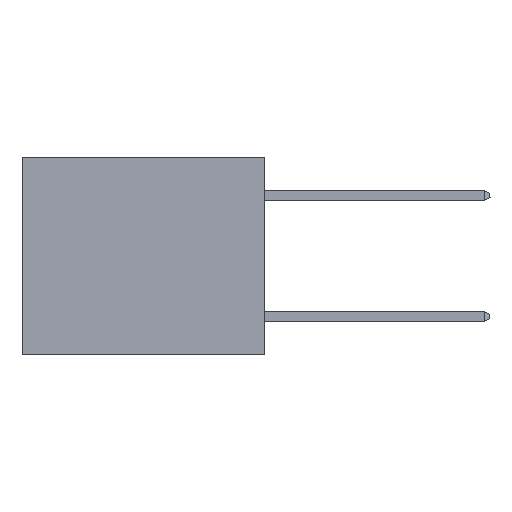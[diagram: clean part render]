
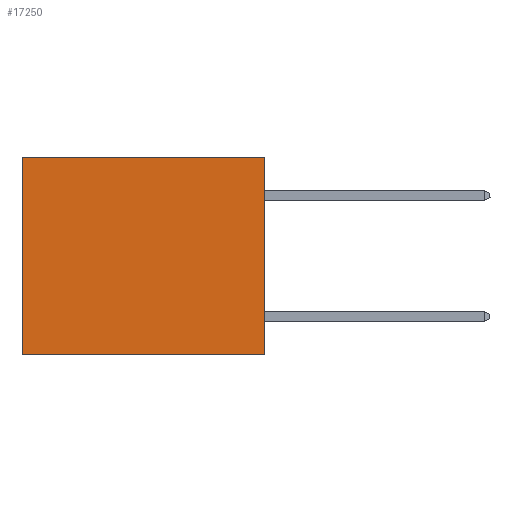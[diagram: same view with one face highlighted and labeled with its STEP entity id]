
A CAD part, left-side view. The second image highlights one B-rep face of the part: STEP entity #17250.
In plain terms, the highlighted planar face has unit normal (-1, 0, 0).
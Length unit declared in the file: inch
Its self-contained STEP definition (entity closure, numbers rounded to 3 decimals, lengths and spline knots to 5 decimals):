
#368 = VECTOR ( 'NONE', #5629, 39.37008 ) ;
#524 = LINE ( 'NONE', #19353, #14289 ) ;
#986 = FACE_OUTER_BOUND ( 'NONE', #22071, .T. ) ;
#1416 = LINE ( 'NONE', #4640, #11259 ) ;
#2075 = CARTESIAN_POINT ( 'NONE',  ( 0.3165, 0., 0. ) ) ;
#3377 = ORIENTED_EDGE ( 'NONE', *, *, #18103, .T. ) ;
#3543 = ORIENTED_EDGE ( 'NONE', *, *, #13408, .F. ) ;
#4015 = DIRECTION ( 'NONE',  ( 0., 0., -1. ) ) ;
#4640 = CARTESIAN_POINT ( 'NONE',  ( 0.3165, 0., -0.49 ) ) ;
#4679 = CARTESIAN_POINT ( 'NONE',  ( 0.3165, 0., 0. ) ) ;
#5357 = ORIENTED_EDGE ( 'NONE', *, *, #7061, .F. ) ;
#5385 = DIRECTION ( 'NONE',  ( 1., 0., 0. ) ) ;
#5629 = DIRECTION ( 'NONE',  ( 0., 1., 0. ) ) ;
#5722 = CARTESIAN_POINT ( 'NONE',  ( 0.3165, 0., -0.49 ) ) ;
#7061 = EDGE_CURVE ( 'NONE', #15803, #22774, #1416, .T. ) ;
#8298 = CARTESIAN_POINT ( 'NONE',  ( 0.3165, 0.6, -0.49 ) ) ;
#9628 = VERTEX_POINT ( 'NONE', #4679 ) ;
#9720 = EDGE_CURVE ( 'NONE', #9628, #15046, #14738, .T. ) ;
#9913 = CARTESIAN_POINT ( 'NONE',  ( 0.3165, 0.6, 0. ) ) ;
#11259 = VECTOR ( 'NONE', #23628, 39.37008 ) ;
#11713 = DIRECTION ( 'NONE',  ( 0., 0., -1. ) ) ;
#12786 = ORIENTED_EDGE ( 'NONE', *, *, #9720, .T. ) ;
#13408 = EDGE_CURVE ( 'NONE', #9628, #15803, #18836, .T. ) ;
#14289 = VECTOR ( 'NONE', #4015, 39.37008 ) ;
#14640 = VECTOR ( 'NONE', #15041, 39.37008 ) ;
#14738 = LINE ( 'NONE', #2075, #368 ) ;
#15041 = DIRECTION ( 'NONE',  ( 0., 0., -1. ) ) ;
#15046 = VERTEX_POINT ( 'NONE', #9913 ) ;
#15803 = VERTEX_POINT ( 'NONE', #5722 ) ;
#16836 = CARTESIAN_POINT ( 'NONE',  ( 0.3165, 0., -0.49 ) ) ;
#17250 = ADVANCED_FACE ( 'NONE', ( #986 ), #24682, .F. ) ;
#18103 = EDGE_CURVE ( 'NONE', #15046, #22774, #524, .T. ) ;
#18836 = LINE ( 'NONE', #18930, #14640 ) ;
#18930 = CARTESIAN_POINT ( 'NONE',  ( 0.3165, 0., -0.49 ) ) ;
#19353 = CARTESIAN_POINT ( 'NONE',  ( 0.3165, 0.6, -0.49 ) ) ;
#20491 = AXIS2_PLACEMENT_3D ( 'NONE', #16836, #5385, #11713 ) ;
#22071 = EDGE_LOOP ( 'NONE', ( #3377, #5357, #3543, #12786 ) ) ;
#22774 = VERTEX_POINT ( 'NONE', #8298 ) ;
#23628 = DIRECTION ( 'NONE',  ( 0., 1., 0. ) ) ;
#24682 = PLANE ( 'NONE',  #20491 ) ;
